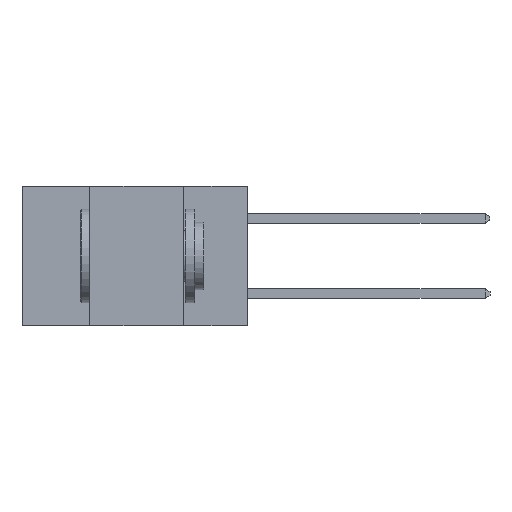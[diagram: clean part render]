
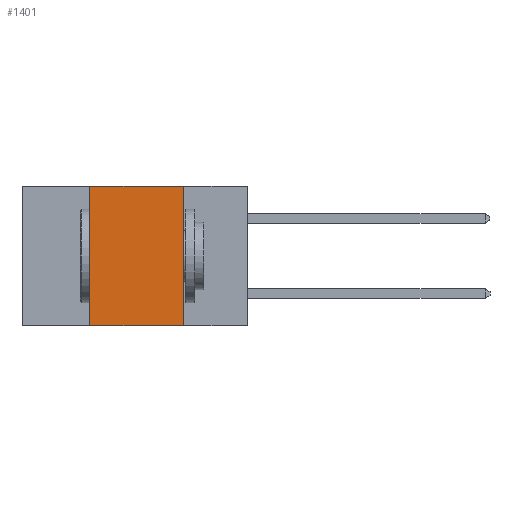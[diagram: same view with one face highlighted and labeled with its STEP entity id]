
A CAD part, left-side view. The second image highlights one B-rep face of the part: STEP entity #1401.
In plain terms, the highlighted planar face has unit normal (-1, 0, 0).
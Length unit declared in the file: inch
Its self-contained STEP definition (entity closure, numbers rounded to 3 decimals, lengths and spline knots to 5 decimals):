
#422 = DIRECTION ( 'NONE',  ( 0., 0., -1. ) ) ;
#454 = VECTOR ( 'NONE', #574, 39.37008 ) ;
#574 = DIRECTION ( 'NONE',  ( 0., -1., 0. ) ) ;
#1018 = ORIENTED_EDGE ( 'NONE', *, *, #8040, .F. ) ;
#1401 = ADVANCED_FACE ( 'NONE', ( #5839 ), #9599, .F. ) ;
#1407 = VECTOR ( 'NONE', #8379, 39.37008 ) ;
#1854 = ORIENTED_EDGE ( 'NONE', *, *, #7061, .F. ) ;
#1904 = DIRECTION ( 'NONE',  ( 1., 0., 0. ) ) ;
#2425 = LINE ( 'NONE', #7349, #454 ) ;
#2884 = CARTESIAN_POINT ( 'NONE',  ( 0., 0.6, 0. ) ) ;
#2962 = VECTOR ( 'NONE', #8430, 39.37008 ) ;
#3160 = EDGE_LOOP ( 'NONE', ( #7174, #1018, #1854, #7591 ) ) ;
#3164 = AXIS2_PLACEMENT_3D ( 'NONE', #2884, #1904, #422 ) ;
#3183 = DIRECTION ( 'NONE',  ( 0., 0., 1. ) ) ;
#3338 = EDGE_CURVE ( 'NONE', #6836, #6446, #10001, .T. ) ;
#3790 = CARTESIAN_POINT ( 'NONE',  ( 0., 0.17, 0. ) ) ;
#3958 = VERTEX_POINT ( 'NONE', #10148 ) ;
#4597 = CARTESIAN_POINT ( 'NONE',  ( 0., 0.17, -0.37 ) ) ;
#5181 = CARTESIAN_POINT ( 'NONE',  ( 0., 0.17, -0.37 ) ) ;
#5268 = LINE ( 'NONE', #4597, #2962 ) ;
#5839 = FACE_OUTER_BOUND ( 'NONE', #3160, .T. ) ;
#6208 = VECTOR ( 'NONE', #3183, 39.37008 ) ;
#6446 = VERTEX_POINT ( 'NONE', #5181 ) ;
#6716 = CARTESIAN_POINT ( 'NONE',  ( 0., 0.6, -0.37 ) ) ;
#6836 = VERTEX_POINT ( 'NONE', #7542 ) ;
#7061 = EDGE_CURVE ( 'NONE', #6836, #3958, #9960, .T. ) ;
#7174 = ORIENTED_EDGE ( 'NONE', *, *, #10825, .F. ) ;
#7349 = CARTESIAN_POINT ( 'NONE',  ( 0., 0.6, 0. ) ) ;
#7542 = CARTESIAN_POINT ( 'NONE',  ( 0., 0.42, -0.37 ) ) ;
#7591 = ORIENTED_EDGE ( 'NONE', *, *, #3338, .T. ) ;
#8040 = EDGE_CURVE ( 'NONE', #3958, #8487, #2425, .T. ) ;
#8379 = DIRECTION ( 'NONE',  ( 0., -1., 0. ) ) ;
#8430 = DIRECTION ( 'NONE',  ( 0., 0., -1. ) ) ;
#8487 = VERTEX_POINT ( 'NONE', #3790 ) ;
#9158 = CARTESIAN_POINT ( 'NONE',  ( 0., 0.42, -0.37 ) ) ;
#9599 = PLANE ( 'NONE',  #3164 ) ;
#9960 = LINE ( 'NONE', #9158, #6208 ) ;
#10001 = LINE ( 'NONE', #6716, #1407 ) ;
#10148 = CARTESIAN_POINT ( 'NONE',  ( 0., 0.42, 0. ) ) ;
#10825 = EDGE_CURVE ( 'NONE', #8487, #6446, #5268, .T. ) ;
